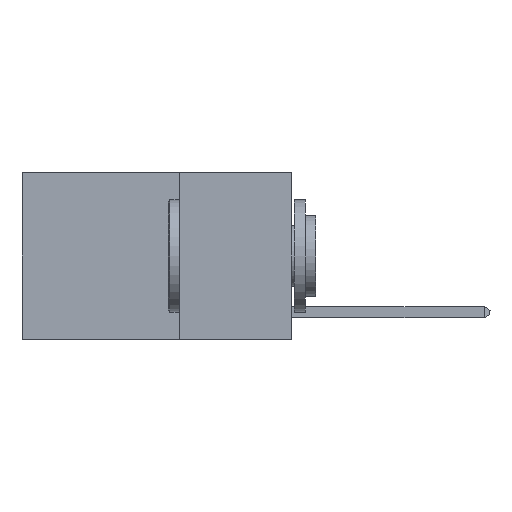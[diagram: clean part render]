
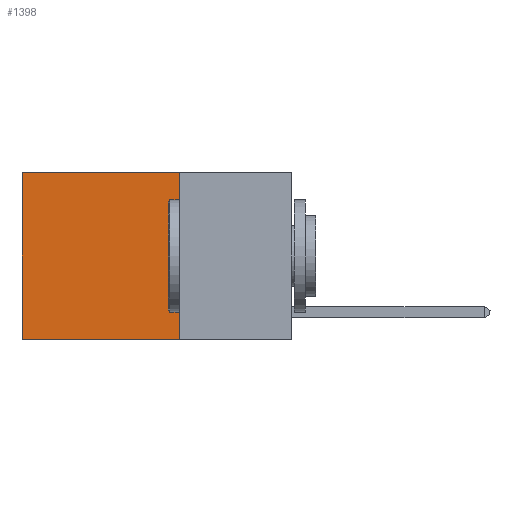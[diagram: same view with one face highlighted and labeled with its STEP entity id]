
A CAD part, left-side view. The second image highlights one B-rep face of the part: STEP entity #1398.
In plain terms, the highlighted planar face has unit normal (-1, 0, 0).
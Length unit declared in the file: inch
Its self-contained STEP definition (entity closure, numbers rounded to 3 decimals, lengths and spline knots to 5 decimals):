
#11 = ORIENTED_EDGE ( 'NONE', *, *, #326, .F. ) ;
#146 = DIRECTION ( 'NONE',  ( 0., 0., -1. ) ) ;
#326 = EDGE_CURVE ( 'NONE', #5365, #9218, #11263, .T. ) ;
#510 = ORIENTED_EDGE ( 'NONE', *, *, #6234, .F. ) ;
#1398 = ADVANCED_FACE ( 'NONE', ( #5467 ), #2675, .F. ) ;
#2081 = AXIS2_PLACEMENT_3D ( 'NONE', #3575, #2605, #2467 ) ;
#2271 = LINE ( 'NONE', #4938, #12321 ) ;
#2306 = EDGE_LOOP ( 'NONE', ( #12018, #510, #11, #9961 ) ) ;
#2467 = DIRECTION ( 'NONE',  ( 0., 0., -1. ) ) ;
#2605 = DIRECTION ( 'NONE',  ( 1., 0., 0. ) ) ;
#2675 = PLANE ( 'NONE',  #2081 ) ;
#2964 = CARTESIAN_POINT ( 'NONE',  ( 0.2625, 0.25, -0.37 ) ) ;
#3575 = CARTESIAN_POINT ( 'NONE',  ( 0.2625, 0.25, 0. ) ) ;
#4523 = CARTESIAN_POINT ( 'NONE',  ( 0.2625, 0.6, 0. ) ) ;
#4582 = VERTEX_POINT ( 'NONE', #5492 ) ;
#4884 = EDGE_CURVE ( 'NONE', #5365, #4582, #2271, .T. ) ;
#4938 = CARTESIAN_POINT ( 'NONE',  ( 0.2625, 0.25, 0. ) ) ;
#5015 = VECTOR ( 'NONE', #8268, 39.37008 ) ;
#5365 = VERTEX_POINT ( 'NONE', #12036 ) ;
#5467 = FACE_OUTER_BOUND ( 'NONE', #2306, .T. ) ;
#5492 = CARTESIAN_POINT ( 'NONE',  ( 0.2625, 0.6, 0. ) ) ;
#5794 = VECTOR ( 'NONE', #11091, 39.37008 ) ;
#5904 = DIRECTION ( 'NONE',  ( 0., 1., 0. ) ) ;
#5941 = VECTOR ( 'NONE', #146, 39.37008 ) ;
#6234 = EDGE_CURVE ( 'NONE', #9218, #11170, #8894, .T. ) ;
#8268 = DIRECTION ( 'NONE',  ( 0., 0., -1. ) ) ;
#8894 = LINE ( 'NONE', #10119, #5794 ) ;
#9218 = VERTEX_POINT ( 'NONE', #2964 ) ;
#9812 = CARTESIAN_POINT ( 'NONE',  ( 0.2625, 0.25, 0. ) ) ;
#9961 = ORIENTED_EDGE ( 'NONE', *, *, #4884, .T. ) ;
#10119 = CARTESIAN_POINT ( 'NONE',  ( 0.2625, 0.25, -0.37 ) ) ;
#10372 = EDGE_CURVE ( 'NONE', #4582, #11170, #10651, .T. ) ;
#10651 = LINE ( 'NONE', #4523, #5015 ) ;
#11091 = DIRECTION ( 'NONE',  ( 0., 1., 0. ) ) ;
#11170 = VERTEX_POINT ( 'NONE', #11978 ) ;
#11263 = LINE ( 'NONE', #9812, #5941 ) ;
#11978 = CARTESIAN_POINT ( 'NONE',  ( 0.2625, 0.6, -0.37 ) ) ;
#12018 = ORIENTED_EDGE ( 'NONE', *, *, #10372, .T. ) ;
#12036 = CARTESIAN_POINT ( 'NONE',  ( 0.2625, 0.25, 0. ) ) ;
#12321 = VECTOR ( 'NONE', #5904, 39.37008 ) ;
